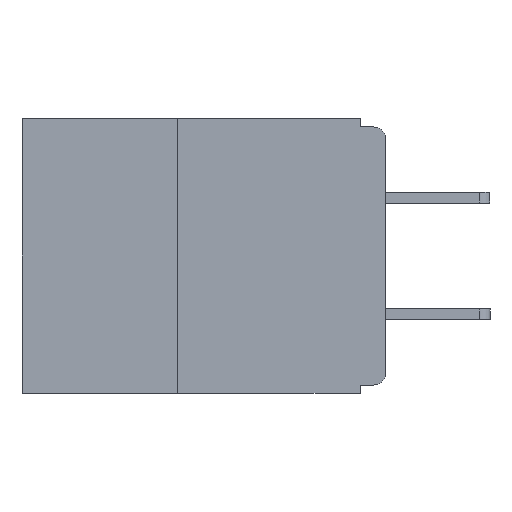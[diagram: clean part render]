
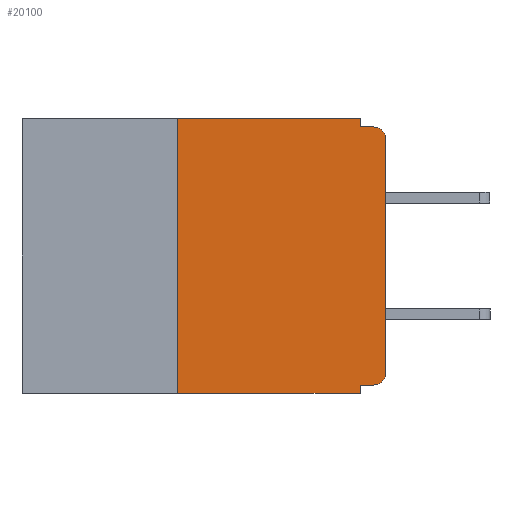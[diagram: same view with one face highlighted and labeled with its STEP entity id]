
A CAD part, left-side view. The second image highlights one B-rep face of the part: STEP entity #20100.
In plain terms, the highlighted planar face has unit normal (-1, 0, 0).
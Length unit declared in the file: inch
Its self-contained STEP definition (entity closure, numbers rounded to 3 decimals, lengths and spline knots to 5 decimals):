
#177 = AXIS2_PLACEMENT_3D ( 'NONE', #4383, #22117, #11511 ) ;
#208 = CARTESIAN_POINT ( 'NONE',  ( 0., 0., -0.025 ) ) ;
#354 = CARTESIAN_POINT ( 'NONE',  ( 0., 0., -0.32 ) ) ;
#382 = LINE ( 'NONE', #16097, #18149 ) ;
#798 = VERTEX_POINT ( 'NONE', #4764 ) ;
#1423 = VECTOR ( 'NONE', #6836, 39.37008 ) ;
#1536 = ORIENTED_EDGE ( 'NONE', *, *, #21694, .T. ) ;
#2092 = CARTESIAN_POINT ( 'NONE',  ( 0., 0.015, -0.32 ) ) ;
#2161 = DIRECTION ( 'NONE',  ( -1., 0., 0. ) ) ;
#2206 = DIRECTION ( 'NONE',  ( 0., 0., -1. ) ) ;
#2328 = CARTESIAN_POINT ( 'NONE',  ( 0., 0.015, -0.305 ) ) ;
#2910 = ORIENTED_EDGE ( 'NONE', *, *, #7029, .T. ) ;
#3285 = EDGE_LOOP ( 'NONE', ( #2910, #12919, #4019, #19282, #21779, #4592, #1536, #3766, #9597, #19387 ) ) ;
#3702 = AXIS2_PLACEMENT_3D ( 'NONE', #2328, #2161, #2206 ) ;
#3704 = EDGE_CURVE ( 'NONE', #7268, #11786, #17683, .T. ) ;
#3766 = ORIENTED_EDGE ( 'NONE', *, *, #13559, .F. ) ;
#4019 = ORIENTED_EDGE ( 'NONE', *, *, #14090, .F. ) ;
#4383 = CARTESIAN_POINT ( 'NONE',  ( 0., 0.437, 0. ) ) ;
#4455 = LINE ( 'NONE', #11981, #18066 ) ;
#4592 = ORIENTED_EDGE ( 'NONE', *, *, #9210, .F. ) ;
#4764 = CARTESIAN_POINT ( 'NONE',  ( 0., 0.031, -0.01 ) ) ;
#5474 = LINE ( 'NONE', #19908, #14894 ) ;
#5754 = LINE ( 'NONE', #354, #14626 ) ;
#5886 = DIRECTION ( 'NONE',  ( 0., 0., -1. ) ) ;
#5924 = CARTESIAN_POINT ( 'NONE',  ( 0., 0.015, -0.025 ) ) ;
#6444 = VERTEX_POINT ( 'NONE', #19292 ) ;
#6836 = DIRECTION ( 'NONE',  ( 0., 0., -1. ) ) ;
#7029 = EDGE_CURVE ( 'NONE', #11786, #17883, #4455, .T. ) ;
#7268 = VERTEX_POINT ( 'NONE', #2092 ) ;
#7272 = CARTESIAN_POINT ( 'NONE',  ( 0., 0.437, -0.33 ) ) ;
#7655 = AXIS2_PLACEMENT_3D ( 'NONE', #5924, #18324, #7679 ) ;
#7679 = DIRECTION ( 'NONE',  ( 0., 0., -1. ) ) ;
#9047 = DIRECTION ( 'NONE',  ( 0., -1., 0. ) ) ;
#9210 = EDGE_CURVE ( 'NONE', #13336, #15139, #5474, .T. ) ;
#9302 = DIRECTION ( 'NONE',  ( 0., 0., 1. ) ) ;
#9597 = ORIENTED_EDGE ( 'NONE', *, *, #12547, .F. ) ;
#9784 = VERTEX_POINT ( 'NONE', #20102 ) ;
#9971 = EDGE_CURVE ( 'NONE', #15139, #15276, #12361, .T. ) ;
#10000 = LINE ( 'NONE', #7272, #18330 ) ;
#10682 = VECTOR ( 'NONE', #5886, 39.37008 ) ;
#10990 = CARTESIAN_POINT ( 'NONE',  ( 0., 0.031, 0. ) ) ;
#11238 = EDGE_CURVE ( 'NONE', #17883, #19923, #13028, .T. ) ;
#11511 = DIRECTION ( 'NONE',  ( 0., 0., -1. ) ) ;
#11786 = VERTEX_POINT ( 'NONE', #16291 ) ;
#11981 = CARTESIAN_POINT ( 'NONE',  ( 0., 0., 0. ) ) ;
#12361 = LINE ( 'NONE', #13629, #13484 ) ;
#12547 = EDGE_CURVE ( 'NONE', #7268, #9784, #5754, .T. ) ;
#12781 = DIRECTION ( 'NONE',  ( 0., 1., 0. ) ) ;
#12919 = ORIENTED_EDGE ( 'NONE', *, *, #11238, .T. ) ;
#13028 = CIRCLE ( 'NONE', #7655, 0.015 ) ;
#13336 = VERTEX_POINT ( 'NONE', #14096 ) ;
#13484 = VECTOR ( 'NONE', #13546, 39.37008 ) ;
#13546 = DIRECTION ( 'NONE',  ( 0., -1., 0. ) ) ;
#13559 = EDGE_CURVE ( 'NONE', #9784, #6444, #20089, .T. ) ;
#13629 = CARTESIAN_POINT ( 'NONE',  ( 0., 0.437, 0. ) ) ;
#13776 = DIRECTION ( 'NONE',  ( 0., 0., 1. ) ) ;
#14090 = EDGE_CURVE ( 'NONE', #798, #19923, #382, .T. ) ;
#14096 = CARTESIAN_POINT ( 'NONE',  ( 0., 0.25, -0.33 ) ) ;
#14297 = DIRECTION ( 'NONE',  ( 0., -1., 0. ) ) ;
#14626 = VECTOR ( 'NONE', #12781, 39.37008 ) ;
#14730 = CARTESIAN_POINT ( 'NONE',  ( 0., 0.031, -0.33 ) ) ;
#14894 = VECTOR ( 'NONE', #9302, 39.37008 ) ;
#15139 = VERTEX_POINT ( 'NONE', #15815 ) ;
#15276 = VERTEX_POINT ( 'NONE', #10990 ) ;
#15596 = LINE ( 'NONE', #22772, #1423 ) ;
#15815 = CARTESIAN_POINT ( 'NONE',  ( 0., 0.25, 0. ) ) ;
#16097 = CARTESIAN_POINT ( 'NONE',  ( 0., 0., -0.01 ) ) ;
#16291 = CARTESIAN_POINT ( 'NONE',  ( 0., 0., -0.305 ) ) ;
#17683 = CIRCLE ( 'NONE', #3702, 0.015 ) ;
#17883 = VERTEX_POINT ( 'NONE', #208 ) ;
#18066 = VECTOR ( 'NONE', #13776, 39.37008 ) ;
#18149 = VECTOR ( 'NONE', #14297, 39.37008 ) ;
#18324 = DIRECTION ( 'NONE',  ( -1., 0., 0. ) ) ;
#18330 = VECTOR ( 'NONE', #9047, 39.37008 ) ;
#18370 = FACE_OUTER_BOUND ( 'NONE', #3285, .T. ) ;
#19282 = ORIENTED_EDGE ( 'NONE', *, *, #20918, .F. ) ;
#19292 = CARTESIAN_POINT ( 'NONE',  ( 0., 0.031, -0.33 ) ) ;
#19387 = ORIENTED_EDGE ( 'NONE', *, *, #3704, .T. ) ;
#19818 = CARTESIAN_POINT ( 'NONE',  ( 0., 0.015, -0.01 ) ) ;
#19908 = CARTESIAN_POINT ( 'NONE',  ( 0., 0.25, -0.33 ) ) ;
#19923 = VERTEX_POINT ( 'NONE', #19818 ) ;
#20089 = LINE ( 'NONE', #14730, #10682 ) ;
#20100 = ADVANCED_FACE ( 'NONE', ( #18370 ), #20332, .F. ) ;
#20102 = CARTESIAN_POINT ( 'NONE',  ( 0., 0.031, -0.32 ) ) ;
#20332 = PLANE ( 'NONE',  #177 ) ;
#20918 = EDGE_CURVE ( 'NONE', #15276, #798, #15596, .T. ) ;
#21694 = EDGE_CURVE ( 'NONE', #13336, #6444, #10000, .T. ) ;
#21779 = ORIENTED_EDGE ( 'NONE', *, *, #9971, .F. ) ;
#22117 = DIRECTION ( 'NONE',  ( 1., 0., 0. ) ) ;
#22772 = CARTESIAN_POINT ( 'NONE',  ( 0., 0.031, 0. ) ) ;
